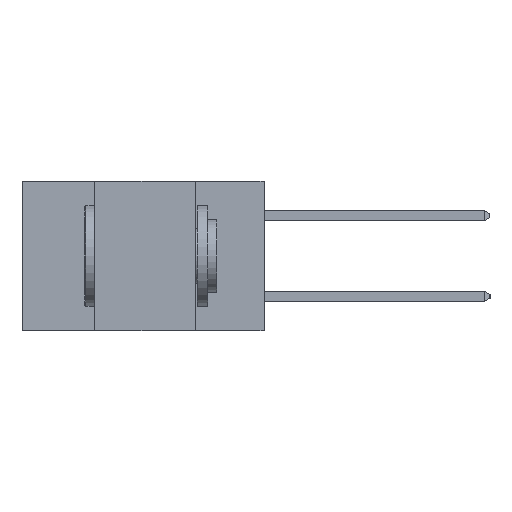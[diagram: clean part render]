
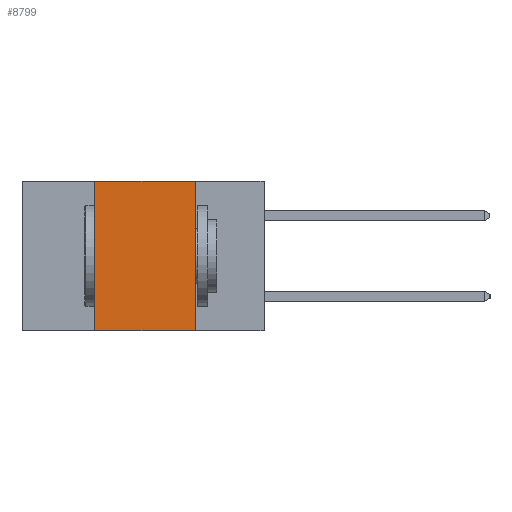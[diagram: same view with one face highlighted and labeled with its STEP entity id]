
A CAD part, left-side view. The second image highlights one B-rep face of the part: STEP entity #8799.
In plain terms, the highlighted planar face has unit normal (-1, 0, 0).
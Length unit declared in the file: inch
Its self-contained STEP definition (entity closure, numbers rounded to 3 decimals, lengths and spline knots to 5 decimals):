
#684 = LINE ( 'NONE', #8998, #4700 ) ;
#719 = EDGE_CURVE ( 'NONE', #4524, #4080, #3095, .T. ) ;
#1609 = LINE ( 'NONE', #5547, #5633 ) ;
#1915 = CARTESIAN_POINT ( 'NONE',  ( 0., 0.17, 0. ) ) ;
#2874 = EDGE_CURVE ( 'NONE', #4080, #6323, #684, .T. ) ;
#3055 = CARTESIAN_POINT ( 'NONE',  ( 0., 0.17, -0.37 ) ) ;
#3095 = LINE ( 'NONE', #6800, #9446 ) ;
#3485 = ORIENTED_EDGE ( 'NONE', *, *, #5950, .T. ) ;
#3506 = PLANE ( 'NONE',  #8064 ) ;
#4080 = VERTEX_POINT ( 'NONE', #1915 ) ;
#4311 = DIRECTION ( 'NONE',  ( 0., 0., -1. ) ) ;
#4524 = VERTEX_POINT ( 'NONE', #9624 ) ;
#4659 = EDGE_LOOP ( 'NONE', ( #6968, #7211, #5344, #3485 ) ) ;
#4700 = VECTOR ( 'NONE', #7700, 39.37008 ) ;
#5344 = ORIENTED_EDGE ( 'NONE', *, *, #7003, .F. ) ;
#5453 = VERTEX_POINT ( 'NONE', #8966 ) ;
#5547 = CARTESIAN_POINT ( 'NONE',  ( 0., 0.6, -0.37 ) ) ;
#5590 = DIRECTION ( 'NONE',  ( 0., -1., 0. ) ) ;
#5633 = VECTOR ( 'NONE', #5590, 39.37008 ) ;
#5950 = EDGE_CURVE ( 'NONE', #5453, #6323, #1609, .T. ) ;
#6231 = VECTOR ( 'NONE', #10039, 39.37008 ) ;
#6323 = VERTEX_POINT ( 'NONE', #3055 ) ;
#6469 = LINE ( 'NONE', #9251, #6231 ) ;
#6800 = CARTESIAN_POINT ( 'NONE',  ( 0., 0.6, 0. ) ) ;
#6968 = ORIENTED_EDGE ( 'NONE', *, *, #2874, .F. ) ;
#7003 = EDGE_CURVE ( 'NONE', #5453, #4524, #6469, .T. ) ;
#7211 = ORIENTED_EDGE ( 'NONE', *, *, #719, .F. ) ;
#7468 = CARTESIAN_POINT ( 'NONE',  ( 0., 0.6, 0. ) ) ;
#7663 = DIRECTION ( 'NONE',  ( 0., -1., 0. ) ) ;
#7700 = DIRECTION ( 'NONE',  ( 0., 0., -1. ) ) ;
#8064 = AXIS2_PLACEMENT_3D ( 'NONE', #7468, #9074, #4311 ) ;
#8799 = ADVANCED_FACE ( 'NONE', ( #9402 ), #3506, .F. ) ;
#8966 = CARTESIAN_POINT ( 'NONE',  ( 0., 0.42, -0.37 ) ) ;
#8998 = CARTESIAN_POINT ( 'NONE',  ( 0., 0.17, -0.37 ) ) ;
#9074 = DIRECTION ( 'NONE',  ( 1., 0., 0. ) ) ;
#9251 = CARTESIAN_POINT ( 'NONE',  ( 0., 0.42, -0.37 ) ) ;
#9402 = FACE_OUTER_BOUND ( 'NONE', #4659, .T. ) ;
#9446 = VECTOR ( 'NONE', #7663, 39.37008 ) ;
#9624 = CARTESIAN_POINT ( 'NONE',  ( 0., 0.42, 0. ) ) ;
#10039 = DIRECTION ( 'NONE',  ( 0., 0., 1. ) ) ;
